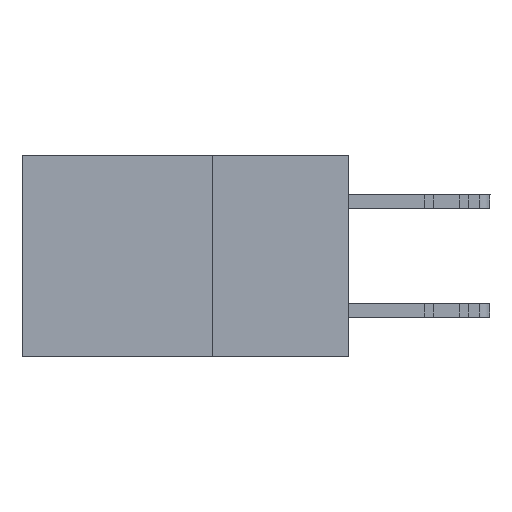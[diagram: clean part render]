
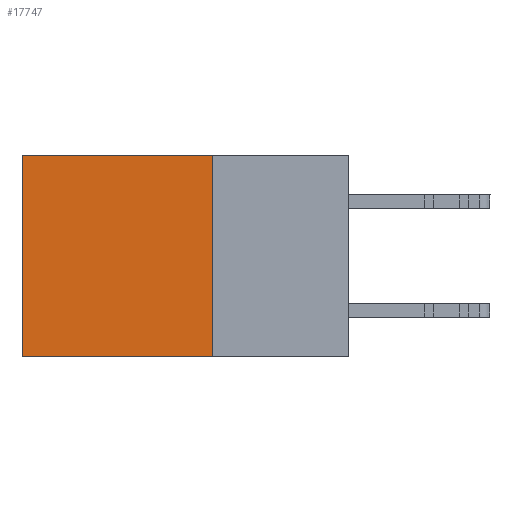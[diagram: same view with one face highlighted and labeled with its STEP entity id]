
A CAD part, left-side view. The second image highlights one B-rep face of the part: STEP entity #17747.
In plain terms, the highlighted planar face has unit normal (-1, 0, 0).
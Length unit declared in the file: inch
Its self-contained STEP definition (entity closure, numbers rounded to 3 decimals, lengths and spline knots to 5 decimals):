
#1841 = VERTEX_POINT ( 'NONE', #7303 ) ;
#2273 = LINE ( 'NONE', #11533, #9800 ) ;
#3547 = VECTOR ( 'NONE', #6632, 39.37008 ) ;
#5189 = ORIENTED_EDGE ( 'NONE', *, *, #13668, .F. ) ;
#5531 = ORIENTED_EDGE ( 'NONE', *, *, #6847, .F. ) ;
#6632 = DIRECTION ( 'NONE',  ( 0., 0., -1. ) ) ;
#6652 = VECTOR ( 'NONE', #17265, 39.37008 ) ;
#6847 = EDGE_CURVE ( 'NONE', #27237, #26110, #17875, .T. ) ;
#7303 = CARTESIAN_POINT ( 'NONE',  ( 0.298, 0.6, 0. ) ) ;
#8253 = EDGE_CURVE ( 'NONE', #1841, #29809, #11640, .T. ) ;
#8611 = CARTESIAN_POINT ( 'NONE',  ( 0.298, 0.25, 0. ) ) ;
#9800 = VECTOR ( 'NONE', #22521, 39.37008 ) ;
#10744 = DIRECTION ( 'NONE',  ( 0., 0., -1. ) ) ;
#11038 = FACE_OUTER_BOUND ( 'NONE', #17288, .T. ) ;
#11533 = CARTESIAN_POINT ( 'NONE',  ( 0.298, 0.25, 0. ) ) ;
#11640 = LINE ( 'NONE', #27866, #3547 ) ;
#13391 = CARTESIAN_POINT ( 'NONE',  ( 0.298, 0.25, 0. ) ) ;
#13456 = DIRECTION ( 'NONE',  ( 1., 0., 0. ) ) ;
#13668 = EDGE_CURVE ( 'NONE', #26110, #29809, #14057, .T. ) ;
#13669 = VECTOR ( 'NONE', #28018, 39.37008 ) ;
#14057 = LINE ( 'NONE', #18629, #13669 ) ;
#15834 = EDGE_CURVE ( 'NONE', #27237, #1841, #2273, .T. ) ;
#17265 = DIRECTION ( 'NONE',  ( 0., 0., -1. ) ) ;
#17288 = EDGE_LOOP ( 'NONE', ( #21889, #5189, #5531, #26800 ) ) ;
#17747 = ADVANCED_FACE ( 'NONE', ( #11038 ), #26967, .F. ) ;
#17875 = LINE ( 'NONE', #19687, #6652 ) ;
#18256 = CARTESIAN_POINT ( 'NONE',  ( 0.298, 0.25, -0.37 ) ) ;
#18629 = CARTESIAN_POINT ( 'NONE',  ( 0.298, 0.25, -0.37 ) ) ;
#19687 = CARTESIAN_POINT ( 'NONE',  ( 0.298, 0.25, 0. ) ) ;
#21889 = ORIENTED_EDGE ( 'NONE', *, *, #8253, .T. ) ;
#22521 = DIRECTION ( 'NONE',  ( 0., 1., 0. ) ) ;
#26110 = VERTEX_POINT ( 'NONE', #18256 ) ;
#26548 = AXIS2_PLACEMENT_3D ( 'NONE', #8611, #13456, #10744 ) ;
#26800 = ORIENTED_EDGE ( 'NONE', *, *, #15834, .T. ) ;
#26967 = PLANE ( 'NONE',  #26548 ) ;
#27237 = VERTEX_POINT ( 'NONE', #13391 ) ;
#27866 = CARTESIAN_POINT ( 'NONE',  ( 0.298, 0.6, 0. ) ) ;
#28018 = DIRECTION ( 'NONE',  ( 0., 1., 0. ) ) ;
#29455 = CARTESIAN_POINT ( 'NONE',  ( 0.298, 0.6, -0.37 ) ) ;
#29809 = VERTEX_POINT ( 'NONE', #29455 ) ;
